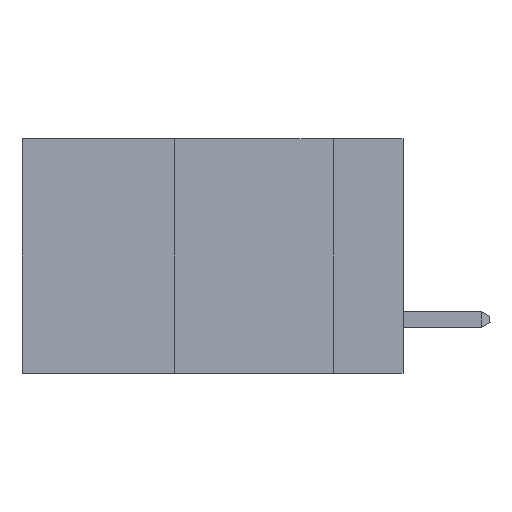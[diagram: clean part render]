
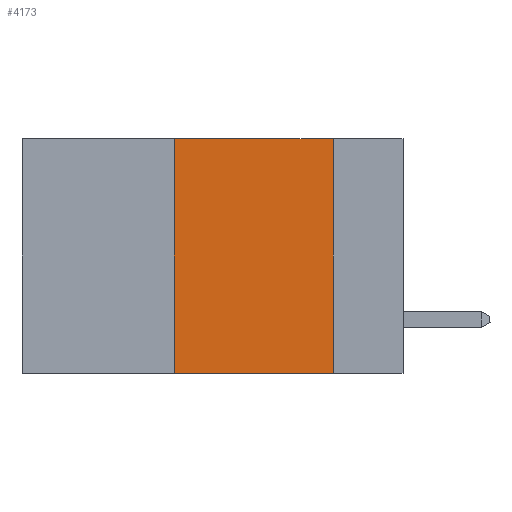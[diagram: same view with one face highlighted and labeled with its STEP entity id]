
A CAD part, left-side view. The second image highlights one B-rep face of the part: STEP entity #4173.
In plain terms, the highlighted planar face has unit normal (-1, 0, 0).
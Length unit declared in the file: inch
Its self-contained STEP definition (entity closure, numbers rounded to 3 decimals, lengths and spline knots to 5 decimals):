
#2061 = ORIENTED_EDGE ( 'NONE', *, *, #20690, .F. ) ;
#2995 = LINE ( 'NONE', #18855, #20325 ) ;
#3160 = VECTOR ( 'NONE', #6432, 39.37008 ) ;
#3415 = PLANE ( 'NONE',  #19852 ) ;
#4173 = ADVANCED_FACE ( 'NONE', ( #20224 ), #3415, .F. ) ;
#4749 = LINE ( 'NONE', #15426, #5431 ) ;
#5431 = VECTOR ( 'NONE', #12674, 39.37008 ) ;
#6225 = CARTESIAN_POINT ( 'NONE',  ( 0., 0.36, 0. ) ) ;
#6432 = DIRECTION ( 'NONE',  ( 0., 0., 1. ) ) ;
#7176 = DIRECTION ( 'NONE',  ( 0., -1., 0. ) ) ;
#8972 = ORIENTED_EDGE ( 'NONE', *, *, #17612, .F. ) ;
#9056 = LINE ( 'NONE', #6225, #3160 ) ;
#9899 = DIRECTION ( 'NONE',  ( 0., 0., -1. ) ) ;
#12453 = EDGE_LOOP ( 'NONE', ( #2061, #25894, #8972, #12986 ) ) ;
#12674 = DIRECTION ( 'NONE',  ( 0., -1., 0. ) ) ;
#12986 = ORIENTED_EDGE ( 'NONE', *, *, #20530, .T. ) ;
#13014 = EDGE_CURVE ( 'NONE', #17340, #14818, #13972, .T. ) ;
#13972 = LINE ( 'NONE', #22707, #26448 ) ;
#14818 = VERTEX_POINT ( 'NONE', #26026 ) ;
#15426 = CARTESIAN_POINT ( 'NONE',  ( 0., 0.6, -0.37 ) ) ;
#17340 = VERTEX_POINT ( 'NONE', #19120 ) ;
#17612 = EDGE_CURVE ( 'NONE', #23368, #17340, #9056, .T. ) ;
#17858 = DIRECTION ( 'NONE',  ( 0., 0., -1. ) ) ;
#18855 = CARTESIAN_POINT ( 'NONE',  ( 0., 0.11, 0. ) ) ;
#19120 = CARTESIAN_POINT ( 'NONE',  ( 0., 0.36, 0. ) ) ;
#19852 = AXIS2_PLACEMENT_3D ( 'NONE', #27679, #23150, #9899 ) ;
#20224 = FACE_OUTER_BOUND ( 'NONE', #12453, .T. ) ;
#20325 = VECTOR ( 'NONE', #17858, 39.37008 ) ;
#20530 = EDGE_CURVE ( 'NONE', #23368, #26031, #4749, .T. ) ;
#20690 = EDGE_CURVE ( 'NONE', #14818, #26031, #2995, .T. ) ;
#22707 = CARTESIAN_POINT ( 'NONE',  ( 0., 0.6, 0. ) ) ;
#23150 = DIRECTION ( 'NONE',  ( 1., 0., 0. ) ) ;
#23368 = VERTEX_POINT ( 'NONE', #26458 ) ;
#25894 = ORIENTED_EDGE ( 'NONE', *, *, #13014, .F. ) ;
#26026 = CARTESIAN_POINT ( 'NONE',  ( 0., 0.11, 0. ) ) ;
#26031 = VERTEX_POINT ( 'NONE', #27862 ) ;
#26448 = VECTOR ( 'NONE', #7176, 39.37008 ) ;
#26458 = CARTESIAN_POINT ( 'NONE',  ( 0., 0.36, -0.37 ) ) ;
#27679 = CARTESIAN_POINT ( 'NONE',  ( 0., 0.6, 0. ) ) ;
#27862 = CARTESIAN_POINT ( 'NONE',  ( 0., 0.11, -0.37 ) ) ;
